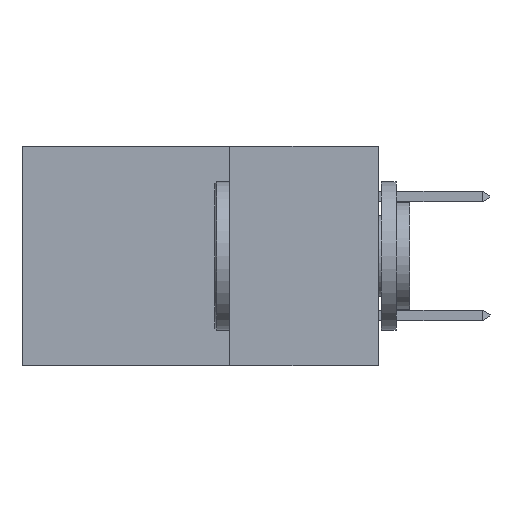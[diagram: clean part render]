
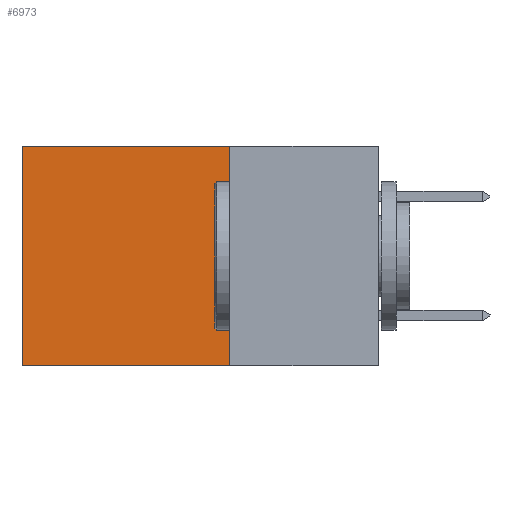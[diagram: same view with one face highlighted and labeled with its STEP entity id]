
A CAD part, left-side view. The second image highlights one B-rep face of the part: STEP entity #6973.
In plain terms, the highlighted planar face has unit normal (-1, 0, 0).
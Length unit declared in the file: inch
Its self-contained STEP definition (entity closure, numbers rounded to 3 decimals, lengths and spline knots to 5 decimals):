
#260 = CARTESIAN_POINT ( 'NONE',  ( 0.2615, 0.6, 0. ) ) ;
#1129 = VERTEX_POINT ( 'NONE', #22308 ) ;
#1888 = LINE ( 'NONE', #12339, #21617 ) ;
#3450 = PLANE ( 'NONE',  #20625 ) ;
#3762 = ORIENTED_EDGE ( 'NONE', *, *, #14046, .T. ) ;
#3865 = LINE ( 'NONE', #15708, #22958 ) ;
#4891 = CARTESIAN_POINT ( 'NONE',  ( 0.2615, 0.25, -0.37 ) ) ;
#5012 = VECTOR ( 'NONE', #8582, 39.37008 ) ;
#5423 = VERTEX_POINT ( 'NONE', #260 ) ;
#6197 = DIRECTION ( 'NONE',  ( 0., 1., 0. ) ) ;
#6649 = EDGE_LOOP ( 'NONE', ( #3762, #24145, #18102, #10192 ) ) ;
#6758 = VERTEX_POINT ( 'NONE', #4891 ) ;
#6973 = ADVANCED_FACE ( 'NONE', ( #14966 ), #3450, .F. ) ;
#8582 = DIRECTION ( 'NONE',  ( 0., 1., 0. ) ) ;
#8696 = VECTOR ( 'NONE', #15066, 39.37008 ) ;
#9274 = DIRECTION ( 'NONE',  ( 1., 0., 0. ) ) ;
#10192 = ORIENTED_EDGE ( 'NONE', *, *, #15637, .T. ) ;
#12339 = CARTESIAN_POINT ( 'NONE',  ( 0.2615, 0.25, -0.37 ) ) ;
#13139 = CARTESIAN_POINT ( 'NONE',  ( 0.2615, 0.6, -0.37 ) ) ;
#14046 = EDGE_CURVE ( 'NONE', #5423, #23472, #14327, .T. ) ;
#14297 = EDGE_CURVE ( 'NONE', #6758, #23472, #3865, .T. ) ;
#14327 = LINE ( 'NONE', #13139, #8696 ) ;
#14577 = CARTESIAN_POINT ( 'NONE',  ( 0.2615, 0.6, -0.37 ) ) ;
#14966 = FACE_OUTER_BOUND ( 'NONE', #6649, .T. ) ;
#15066 = DIRECTION ( 'NONE',  ( 0., 0., -1. ) ) ;
#15637 = EDGE_CURVE ( 'NONE', #1129, #5423, #19096, .T. ) ;
#15708 = CARTESIAN_POINT ( 'NONE',  ( 0.2615, 0.25, -0.37 ) ) ;
#17083 = EDGE_CURVE ( 'NONE', #1129, #6758, #1888, .T. ) ;
#18097 = CARTESIAN_POINT ( 'NONE',  ( 0.2615, 0.25, 0. ) ) ;
#18102 = ORIENTED_EDGE ( 'NONE', *, *, #17083, .F. ) ;
#19096 = LINE ( 'NONE', #18097, #5012 ) ;
#20625 = AXIS2_PLACEMENT_3D ( 'NONE', #20678, #9274, #22552 ) ;
#20678 = CARTESIAN_POINT ( 'NONE',  ( 0.2615, 0.25, -0.37 ) ) ;
#21617 = VECTOR ( 'NONE', #23804, 39.37008 ) ;
#22308 = CARTESIAN_POINT ( 'NONE',  ( 0.2615, 0.25, 0. ) ) ;
#22552 = DIRECTION ( 'NONE',  ( 0., 0., -1. ) ) ;
#22958 = VECTOR ( 'NONE', #6197, 39.37008 ) ;
#23472 = VERTEX_POINT ( 'NONE', #14577 ) ;
#23804 = DIRECTION ( 'NONE',  ( 0., 0., -1. ) ) ;
#24145 = ORIENTED_EDGE ( 'NONE', *, *, #14297, .F. ) ;
